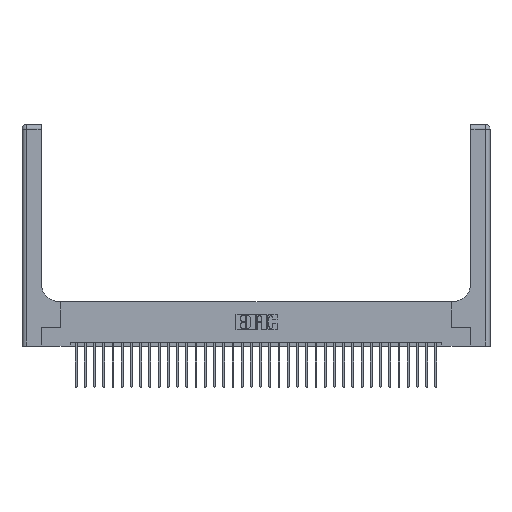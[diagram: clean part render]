
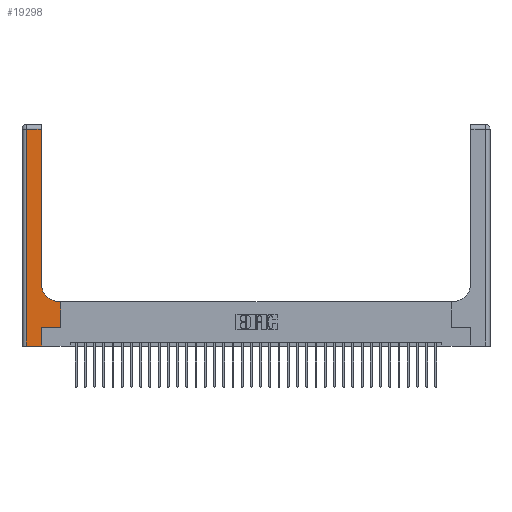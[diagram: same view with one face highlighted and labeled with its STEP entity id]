
A CAD part, top view. The second image highlights one B-rep face of the part: STEP entity #19298.
In plain terms, the highlighted planar face has unit normal (0, 0, 1).
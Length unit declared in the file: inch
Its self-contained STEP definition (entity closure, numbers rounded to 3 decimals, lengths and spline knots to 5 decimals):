
#384 = VERTEX_POINT ( 'NONE', #24990 ) ;
#710 = DIRECTION ( 'NONE',  ( -1., 0., 0. ) ) ;
#989 = VECTOR ( 'NONE', #31400, 39.37008 ) ;
#1802 = FACE_OUTER_BOUND ( 'NONE', #12313, .T. ) ;
#1989 = EDGE_CURVE ( 'NONE', #6272, #15054, #5657, .T. ) ;
#2579 = ORIENTED_EDGE ( 'NONE', *, *, #23951, .T. ) ;
#3085 = PLANE ( 'NONE',  #27741 ) ;
#3168 = EDGE_CURVE ( 'NONE', #384, #22905, #12749, .T. ) ;
#3222 = DIRECTION ( 'NONE',  ( -1., 0., 0. ) ) ;
#3246 = VERTEX_POINT ( 'NONE', #23713 ) ;
#4045 = LINE ( 'NONE', #21982, #20789 ) ;
#4398 = CARTESIAN_POINT ( 'NONE',  ( 0.51, 0.85, 0.37 ) ) ;
#4676 = CARTESIAN_POINT ( 'NONE',  ( 0.528, 0.25, 0.37 ) ) ;
#5657 = LINE ( 'NONE', #6650, #11383 ) ;
#5819 = VERTEX_POINT ( 'NONE', #28595 ) ;
#6272 = VERTEX_POINT ( 'NONE', #20845 ) ;
#6650 = CARTESIAN_POINT ( 'NONE',  ( 0.265, 0., 0.37 ) ) ;
#7084 = ORIENTED_EDGE ( 'NONE', *, *, #3168, .T. ) ;
#7511 = CARTESIAN_POINT ( 'NONE',  ( 0.06, 0., 0.37 ) ) ;
#7736 = LINE ( 'NONE', #22269, #13443 ) ;
#7861 = DIRECTION ( 'NONE',  ( 0., 0., -1. ) ) ;
#8532 = ORIENTED_EDGE ( 'NONE', *, *, #15285, .T. ) ;
#8954 = VERTEX_POINT ( 'NONE', #4676 ) ;
#9216 = CARTESIAN_POINT ( 'NONE',  ( 0., 2.94, 0.37 ) ) ;
#9939 = EDGE_CURVE ( 'NONE', #22905, #6272, #19618, .T. ) ;
#11383 = VECTOR ( 'NONE', #30964, 39.37008 ) ;
#12313 = EDGE_LOOP ( 'NONE', ( #24154, #8532, #7084, #29008, #31531, #23155, #28810, #18553, #2579 ) ) ;
#12749 = LINE ( 'NONE', #18591, #26107 ) ;
#13443 = VECTOR ( 'NONE', #3222, 39.37008 ) ;
#13664 = LINE ( 'NONE', #24868, #22030 ) ;
#14330 = VERTEX_POINT ( 'NONE', #27277 ) ;
#15054 = VERTEX_POINT ( 'NONE', #20790 ) ;
#15096 = CIRCLE ( 'NONE', #17452, 0.25 ) ;
#15215 = DIRECTION ( 'NONE',  ( 1., 0., 0. ) ) ;
#15285 = EDGE_CURVE ( 'NONE', #3246, #384, #26934, .T. ) ;
#17452 = AXIS2_PLACEMENT_3D ( 'NONE', #4398, #30933, #19173 ) ;
#18553 = ORIENTED_EDGE ( 'NONE', *, *, #26461, .T. ) ;
#18591 = CARTESIAN_POINT ( 'NONE',  ( 0.06, 3., 0.37 ) ) ;
#18640 = EDGE_CURVE ( 'NONE', #15054, #8954, #13664, .T. ) ;
#19173 = DIRECTION ( 'NONE',  ( 1., 0., 0. ) ) ;
#19298 = ADVANCED_FACE ( 'NONE', ( #1802 ), #3085, .F. ) ;
#19618 = LINE ( 'NONE', #29022, #26867 ) ;
#19758 = DIRECTION ( 'NONE',  ( 0., 1., 0. ) ) ;
#19844 = DIRECTION ( 'NONE',  ( 0., 1., 0. ) ) ;
#19886 = EDGE_CURVE ( 'NONE', #21043, #3246, #4045, .T. ) ;
#20789 = VECTOR ( 'NONE', #19758, 39.37008 ) ;
#20790 = CARTESIAN_POINT ( 'NONE',  ( 0.265, 0.25, 0.37 ) ) ;
#20822 = DIRECTION ( 'NONE',  ( 0., -1., 0. ) ) ;
#20845 = CARTESIAN_POINT ( 'NONE',  ( 0.265, 0., 0.37 ) ) ;
#21043 = VERTEX_POINT ( 'NONE', #22018 ) ;
#21982 = CARTESIAN_POINT ( 'NONE',  ( 0.26, 3., 0.37 ) ) ;
#22018 = CARTESIAN_POINT ( 'NONE',  ( 0.26, 0.85, 0.37 ) ) ;
#22030 = VECTOR ( 'NONE', #27017, 39.37008 ) ;
#22269 = CARTESIAN_POINT ( 'NONE',  ( 0.26, 0.6, 0.37 ) ) ;
#22541 = CARTESIAN_POINT ( 'NONE',  ( 0., 3., 0.37 ) ) ;
#22593 = LINE ( 'NONE', #26898, #24905 ) ;
#22905 = VERTEX_POINT ( 'NONE', #7511 ) ;
#23155 = ORIENTED_EDGE ( 'NONE', *, *, #18640, .T. ) ;
#23713 = CARTESIAN_POINT ( 'NONE',  ( 0.26, 2.94, 0.37 ) ) ;
#23951 = EDGE_CURVE ( 'NONE', #5819, #21043, #15096, .T. ) ;
#24154 = ORIENTED_EDGE ( 'NONE', *, *, #19886, .T. ) ;
#24868 = CARTESIAN_POINT ( 'NONE',  ( 0.265, 0.25, 0.37 ) ) ;
#24905 = VECTOR ( 'NONE', #19844, 39.37008 ) ;
#24990 = CARTESIAN_POINT ( 'NONE',  ( 0.06, 2.94, 0.37 ) ) ;
#25882 = EDGE_CURVE ( 'NONE', #8954, #14330, #22593, .T. ) ;
#26107 = VECTOR ( 'NONE', #20822, 39.37008 ) ;
#26461 = EDGE_CURVE ( 'NONE', #14330, #5819, #7736, .T. ) ;
#26867 = VECTOR ( 'NONE', #15215, 39.37008 ) ;
#26898 = CARTESIAN_POINT ( 'NONE',  ( 0.528, 0.25, 0.37 ) ) ;
#26934 = LINE ( 'NONE', #9216, #989 ) ;
#27017 = DIRECTION ( 'NONE',  ( 1., 0., 0. ) ) ;
#27277 = CARTESIAN_POINT ( 'NONE',  ( 0.528, 0.6, 0.37 ) ) ;
#27741 = AXIS2_PLACEMENT_3D ( 'NONE', #22541, #7861, #710 ) ;
#28595 = CARTESIAN_POINT ( 'NONE',  ( 0.51, 0.6, 0.37 ) ) ;
#28810 = ORIENTED_EDGE ( 'NONE', *, *, #25882, .T. ) ;
#29008 = ORIENTED_EDGE ( 'NONE', *, *, #9939, .T. ) ;
#29022 = CARTESIAN_POINT ( 'NONE',  ( 0., 0., 0.37 ) ) ;
#30933 = DIRECTION ( 'NONE',  ( 0., 0., -1. ) ) ;
#30964 = DIRECTION ( 'NONE',  ( 0., 1., 0. ) ) ;
#31400 = DIRECTION ( 'NONE',  ( -1., 0., 0. ) ) ;
#31531 = ORIENTED_EDGE ( 'NONE', *, *, #1989, .T. ) ;
